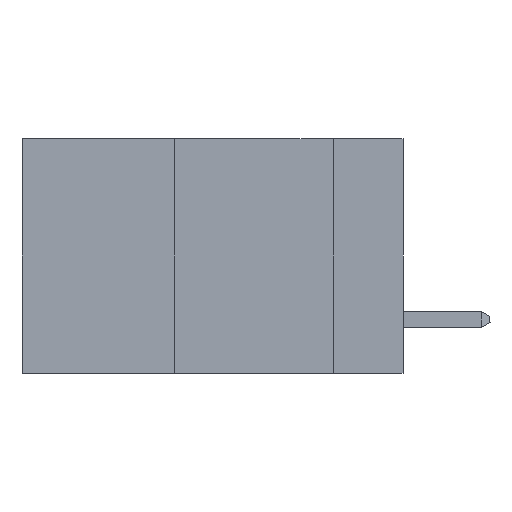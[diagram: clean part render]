
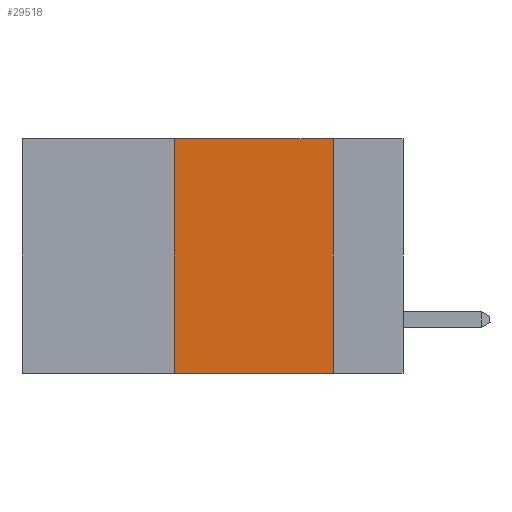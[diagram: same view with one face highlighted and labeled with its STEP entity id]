
A CAD part, left-side view. The second image highlights one B-rep face of the part: STEP entity #29518.
In plain terms, the highlighted planar face has unit normal (-1, 0, 0).
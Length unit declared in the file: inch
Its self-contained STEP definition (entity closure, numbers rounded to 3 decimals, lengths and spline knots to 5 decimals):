
#125 = AXIS2_PLACEMENT_3D ( 'NONE', #1792, #2200, #23261 ) ;
#777 = LINE ( 'NONE', #24477, #20465 ) ;
#1340 = EDGE_LOOP ( 'NONE', ( #14586, #12338, #23952, #34309 ) ) ;
#1792 = CARTESIAN_POINT ( 'NONE',  ( 0., 0.6, 0. ) ) ;
#1829 = EDGE_CURVE ( 'NONE', #6079, #4137, #34202, .T. ) ;
#2200 = DIRECTION ( 'NONE',  ( 1., 0., 0. ) ) ;
#3321 = VECTOR ( 'NONE', #22637, 39.37008 ) ;
#4137 = VERTEX_POINT ( 'NONE', #37690 ) ;
#6079 = VERTEX_POINT ( 'NONE', #35748 ) ;
#6094 = VERTEX_POINT ( 'NONE', #32950 ) ;
#6991 = DIRECTION ( 'NONE',  ( 0., -1., 0. ) ) ;
#7205 = CARTESIAN_POINT ( 'NONE',  ( 0., 0.6, -0.37 ) ) ;
#8947 = DIRECTION ( 'NONE',  ( 0., -1., 0. ) ) ;
#9348 = CARTESIAN_POINT ( 'NONE',  ( 0., 0.6, 0. ) ) ;
#11829 = DIRECTION ( 'NONE',  ( 0., 0., -1. ) ) ;
#12338 = ORIENTED_EDGE ( 'NONE', *, *, #1829, .F. ) ;
#12593 = EDGE_CURVE ( 'NONE', #38062, #6094, #34440, .T. ) ;
#13080 = CARTESIAN_POINT ( 'NONE',  ( 0., 0.36, -0.37 ) ) ;
#14004 = PLANE ( 'NONE',  #125 ) ;
#14586 = ORIENTED_EDGE ( 'NONE', *, *, #34518, .F. ) ;
#19427 = LINE ( 'NONE', #31655, #3321 ) ;
#20465 = VECTOR ( 'NONE', #11829, 39.37008 ) ;
#22637 = DIRECTION ( 'NONE',  ( 0., 0., 1. ) ) ;
#22812 = VECTOR ( 'NONE', #8947, 39.37008 ) ;
#23261 = DIRECTION ( 'NONE',  ( 0., 0., -1. ) ) ;
#23952 = ORIENTED_EDGE ( 'NONE', *, *, #31089, .F. ) ;
#24477 = CARTESIAN_POINT ( 'NONE',  ( 0., 0.11, 0. ) ) ;
#29518 = ADVANCED_FACE ( 'NONE', ( #38665 ), #14004, .F. ) ;
#31089 = EDGE_CURVE ( 'NONE', #38062, #6079, #19427, .T. ) ;
#31655 = CARTESIAN_POINT ( 'NONE',  ( 0., 0.36, 0. ) ) ;
#32950 = CARTESIAN_POINT ( 'NONE',  ( 0., 0.11, -0.37 ) ) ;
#34202 = LINE ( 'NONE', #9348, #22812 ) ;
#34309 = ORIENTED_EDGE ( 'NONE', *, *, #12593, .T. ) ;
#34440 = LINE ( 'NONE', #7205, #35129 ) ;
#34518 = EDGE_CURVE ( 'NONE', #4137, #6094, #777, .T. ) ;
#35129 = VECTOR ( 'NONE', #6991, 39.37008 ) ;
#35748 = CARTESIAN_POINT ( 'NONE',  ( 0., 0.36, 0. ) ) ;
#37690 = CARTESIAN_POINT ( 'NONE',  ( 0., 0.11, 0. ) ) ;
#38062 = VERTEX_POINT ( 'NONE', #13080 ) ;
#38665 = FACE_OUTER_BOUND ( 'NONE', #1340, .T. ) ;
